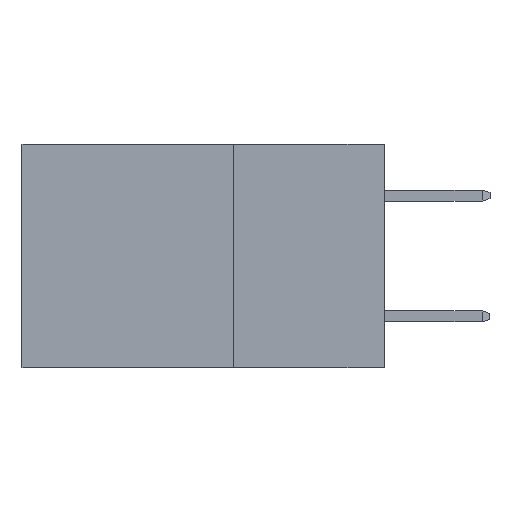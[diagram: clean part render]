
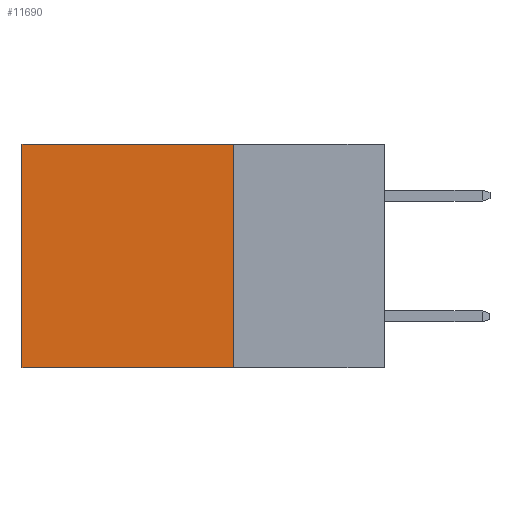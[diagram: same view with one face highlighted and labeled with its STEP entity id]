
A CAD part, left-side view. The second image highlights one B-rep face of the part: STEP entity #11690.
In plain terms, the highlighted planar face has unit normal (-1, 0, 0).
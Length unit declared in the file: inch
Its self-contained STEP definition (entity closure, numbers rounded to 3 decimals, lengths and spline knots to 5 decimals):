
#475 = DIRECTION ( 'NONE',  ( 0., 1., 0. ) ) ;
#1820 = DIRECTION ( 'NONE',  ( 0., 0., -1. ) ) ;
#2610 = LINE ( 'NONE', #6531, #22120 ) ;
#2857 = VERTEX_POINT ( 'NONE', #16202 ) ;
#3000 = CARTESIAN_POINT ( 'NONE',  ( 0.298, 0.25, 0. ) ) ;
#4251 = ORIENTED_EDGE ( 'NONE', *, *, #16397, .T. ) ;
#4847 = VERTEX_POINT ( 'NONE', #12108 ) ;
#5653 = DIRECTION ( 'NONE',  ( 1., 0., 0. ) ) ;
#5894 = VECTOR ( 'NONE', #1820, 39.37008 ) ;
#6531 = CARTESIAN_POINT ( 'NONE',  ( 0.298, 0.6, 0. ) ) ;
#7599 = VERTEX_POINT ( 'NONE', #30608 ) ;
#7690 = EDGE_LOOP ( 'NONE', ( #22341, #14814, #21716, #4251 ) ) ;
#8791 = CARTESIAN_POINT ( 'NONE',  ( 0.298, 0.25, -0.37 ) ) ;
#9252 = EDGE_CURVE ( 'NONE', #4847, #21114, #12722, .T. ) ;
#11414 = DIRECTION ( 'NONE',  ( 0., 1., 0. ) ) ;
#11690 = ADVANCED_FACE ( 'NONE', ( #28816 ), #15813, .F. ) ;
#12108 = CARTESIAN_POINT ( 'NONE',  ( 0.298, 0.25, 0. ) ) ;
#12722 = LINE ( 'NONE', #17203, #5894 ) ;
#12868 = LINE ( 'NONE', #8791, #31804 ) ;
#13304 = AXIS2_PLACEMENT_3D ( 'NONE', #3000, #5653, #23317 ) ;
#14814 = ORIENTED_EDGE ( 'NONE', *, *, #32286, .F. ) ;
#15813 = PLANE ( 'NONE',  #13304 ) ;
#16202 = CARTESIAN_POINT ( 'NONE',  ( 0.298, 0.6, 0. ) ) ;
#16397 = EDGE_CURVE ( 'NONE', #4847, #2857, #27871, .T. ) ;
#17203 = CARTESIAN_POINT ( 'NONE',  ( 0.298, 0.25, 0. ) ) ;
#17453 = EDGE_CURVE ( 'NONE', #2857, #7599, #2610, .T. ) ;
#18425 = CARTESIAN_POINT ( 'NONE',  ( 0.298, 0.25, 0. ) ) ;
#21114 = VERTEX_POINT ( 'NONE', #31077 ) ;
#21716 = ORIENTED_EDGE ( 'NONE', *, *, #9252, .F. ) ;
#22120 = VECTOR ( 'NONE', #26590, 39.37008 ) ;
#22341 = ORIENTED_EDGE ( 'NONE', *, *, #17453, .T. ) ;
#23317 = DIRECTION ( 'NONE',  ( 0., 0., -1. ) ) ;
#26342 = VECTOR ( 'NONE', #475, 39.37008 ) ;
#26590 = DIRECTION ( 'NONE',  ( 0., 0., -1. ) ) ;
#27871 = LINE ( 'NONE', #18425, #26342 ) ;
#28816 = FACE_OUTER_BOUND ( 'NONE', #7690, .T. ) ;
#30608 = CARTESIAN_POINT ( 'NONE',  ( 0.298, 0.6, -0.37 ) ) ;
#31077 = CARTESIAN_POINT ( 'NONE',  ( 0.298, 0.25, -0.37 ) ) ;
#31804 = VECTOR ( 'NONE', #11414, 39.37008 ) ;
#32286 = EDGE_CURVE ( 'NONE', #21114, #7599, #12868, .T. ) ;
